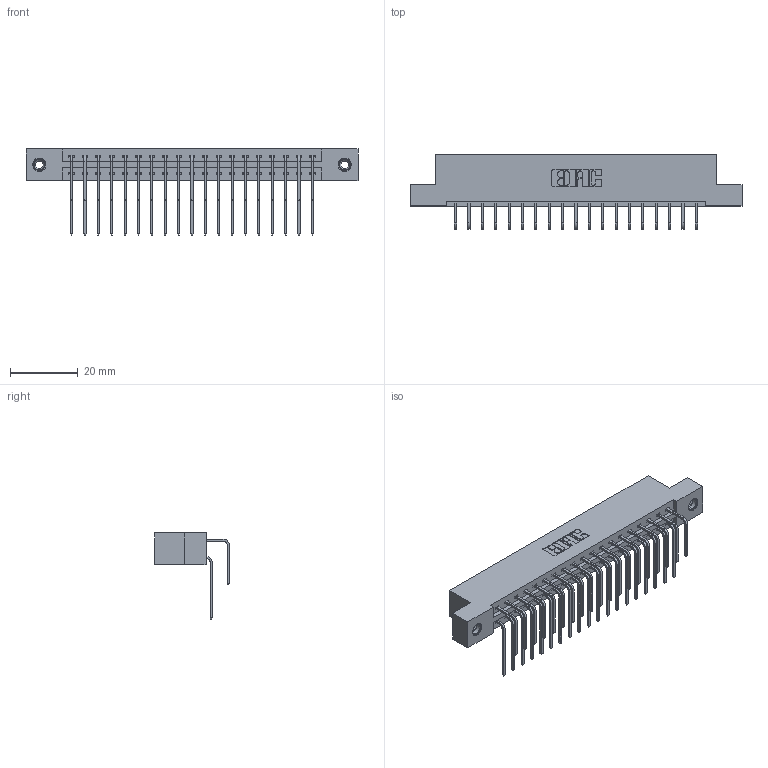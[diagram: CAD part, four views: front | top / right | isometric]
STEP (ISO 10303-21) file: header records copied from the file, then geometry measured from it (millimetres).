
FILE_DESCRIPTION (( 'STEP AP203' ), '1' );
FILE_NAME ('387-038-558-208.STEP', '2018-09-19T06:36:56', ( '' ), ( '' ), 'SwSTEP 2.0', 'SolidWorks 2016', '' );
FILE_SCHEMA (( 'CONFIG_CONTROL_DESIGN' ));
Length unit declared in the file: inch
Products named in the file (5): 345-292-001_558 Tail - 2; 345-250-001_345-250-003-102; 387-038-558-208; 337 Part_Flush Mounting Lugs - 0.156 Dia-TI; 345-292-001_558 559 Tail - 1
Assembly tree (41 placements, depth 2):
  387-038-558-208
    337 Part_Flush Mounting Lugs - 0.156 Dia-TI
    345-292-001_558 559 Tail - 1  x19
    345-292-001_558 Tail - 2  x19
    345-250-001_345-250-003-102  x2
Bounding box: 98.3 x 22.17 x 25.53 mm (x, y, z)
Volume: 10266 mm3; surface area: 12506.9 mm2
Topology: 41 solids, 41 shells, 2302 faces, 6793 edges, 4470 vertices
Faces by surface type: plane 1622, cylinder 664, cone 12, torus 4
Entity records: 20676 total; most frequent: CARTESIAN_POINT 3528, ORIENTED_EDGE 3406, DIRECTION 3057, EDGE_CURVE 1703, VECTOR 1515, LINE 1515, VERTEX_POINT 1128, AXIS2_PLACEMENT_3D 771
